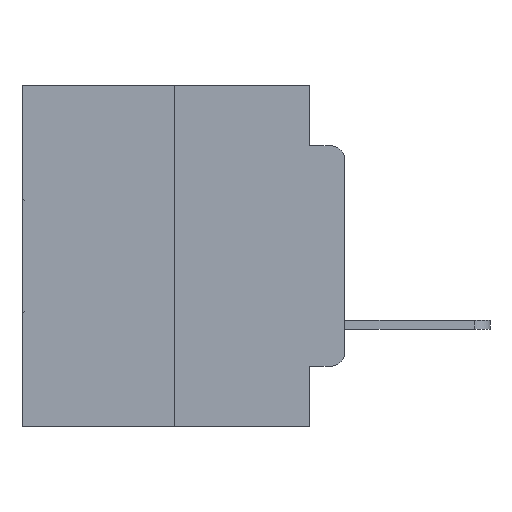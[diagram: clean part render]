
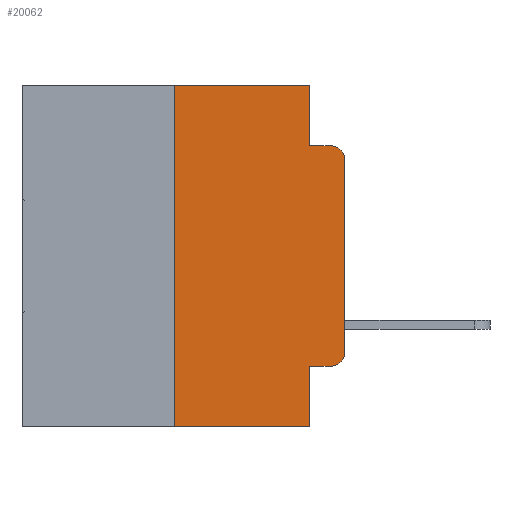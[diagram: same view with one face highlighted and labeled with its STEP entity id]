
A CAD part, left-side view. The second image highlights one B-rep face of the part: STEP entity #20062.
In plain terms, the highlighted planar face has unit normal (-1, 0, 0).
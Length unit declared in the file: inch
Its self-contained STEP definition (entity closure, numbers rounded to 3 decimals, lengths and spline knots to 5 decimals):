
#60 = CARTESIAN_POINT ( 'NONE',  ( 0., 0.051, -0.0885 ) ) ;
#157 = CARTESIAN_POINT ( 'NONE',  ( 0., 0.02, -0.3915 ) ) ;
#269 = ORIENTED_EDGE ( 'NONE', *, *, #30994, .F. ) ;
#780 = LINE ( 'NONE', #2235, #20785 ) ;
#942 = CARTESIAN_POINT ( 'NONE',  ( 0., 0., -0.1085 ) ) ;
#957 = ORIENTED_EDGE ( 'NONE', *, *, #22711, .T. ) ;
#1211 = ORIENTED_EDGE ( 'NONE', *, *, #21705, .T. ) ;
#1586 = VECTOR ( 'NONE', #13618, 39.37008 ) ;
#1912 = VERTEX_POINT ( 'NONE', #25877 ) ;
#2235 = CARTESIAN_POINT ( 'NONE',  ( 0., 0.051, -0.4115 ) ) ;
#2318 = EDGE_CURVE ( 'NONE', #24108, #1912, #25616, .T. ) ;
#2443 = VECTOR ( 'NONE', #11772, 39.37008 ) ;
#2888 = DIRECTION ( 'NONE',  ( 0., 0., -1. ) ) ;
#3229 = CARTESIAN_POINT ( 'NONE',  ( 0., 0.02, -0.4115 ) ) ;
#3247 = LINE ( 'NONE', #16661, #28120 ) ;
#4079 = VECTOR ( 'NONE', #18414, 39.37008 ) ;
#4267 = EDGE_CURVE ( 'NONE', #18400, #5257, #29438, .T. ) ;
#5257 = VERTEX_POINT ( 'NONE', #10855 ) ;
#5458 = CARTESIAN_POINT ( 'NONE',  ( 0., 0.051, -0.4115 ) ) ;
#5983 = PLANE ( 'NONE',  #12630 ) ;
#6089 = AXIS2_PLACEMENT_3D ( 'NONE', #24161, #29414, #29419 ) ;
#6649 = VECTOR ( 'NONE', #28422, 39.37008 ) ;
#6708 = CARTESIAN_POINT ( 'NONE',  ( 0., 0., -0.3915 ) ) ;
#7072 = CARTESIAN_POINT ( 'NONE',  ( 0., 0.25, -0.5 ) ) ;
#7137 = CARTESIAN_POINT ( 'NONE',  ( 0., 0.051, -0.0885 ) ) ;
#7579 = VERTEX_POINT ( 'NONE', #5458 ) ;
#7783 = AXIS2_PLACEMENT_3D ( 'NONE', #157, #18038, #2888 ) ;
#8531 = DIRECTION ( 'NONE',  ( 0., 0., -1. ) ) ;
#8793 = VERTEX_POINT ( 'NONE', #6708 ) ;
#10855 = CARTESIAN_POINT ( 'NONE',  ( 0., 0.25, 0. ) ) ;
#11091 = DIRECTION ( 'NONE',  ( 0., 0., -1. ) ) ;
#11772 = DIRECTION ( 'NONE',  ( 0., -1., 0. ) ) ;
#12368 = VERTEX_POINT ( 'NONE', #21051 ) ;
#12630 = AXIS2_PLACEMENT_3D ( 'NONE', #22774, #25169, #11091 ) ;
#13618 = DIRECTION ( 'NONE',  ( 0., 0., 1. ) ) ;
#13876 = LINE ( 'NONE', #16652, #19439 ) ;
#14248 = DIRECTION ( 'NONE',  ( 0., 0., -1. ) ) ;
#15031 = EDGE_CURVE ( 'NONE', #17494, #1912, #26417, .T. ) ;
#16448 = EDGE_CURVE ( 'NONE', #12368, #17494, #3247, .T. ) ;
#16652 = CARTESIAN_POINT ( 'NONE',  ( 0., 0.473, 0. ) ) ;
#16661 = CARTESIAN_POINT ( 'NONE',  ( 0., 0.051, 0. ) ) ;
#17494 = VERTEX_POINT ( 'NONE', #60 ) ;
#17636 = EDGE_LOOP ( 'NONE', ( #18782, #19552, #21857, #22356, #22534, #23887, #26250, #269, #957, #1211 ) ) ;
#18038 = DIRECTION ( 'NONE',  ( -1., 0., 0. ) ) ;
#18062 = EDGE_CURVE ( 'NONE', #8793, #24108, #31083, .T. ) ;
#18400 = VERTEX_POINT ( 'NONE', #7072 ) ;
#18414 = DIRECTION ( 'NONE',  ( 0., 0., 1. ) ) ;
#18616 = CARTESIAN_POINT ( 'NONE',  ( 0., 0.25, 0. ) ) ;
#18782 = ORIENTED_EDGE ( 'NONE', *, *, #18062, .T. ) ;
#18918 = CARTESIAN_POINT ( 'NONE',  ( 0., 0.051, -0.5 ) ) ;
#19439 = VECTOR ( 'NONE', #25855, 39.37008 ) ;
#19552 = ORIENTED_EDGE ( 'NONE', *, *, #2318, .T. ) ;
#19797 = CIRCLE ( 'NONE', #7783, 0.02 ) ;
#20062 = ADVANCED_FACE ( 'NONE', ( #20958 ), #5983, .F. ) ;
#20069 = VERTEX_POINT ( 'NONE', #3229 ) ;
#20231 = VERTEX_POINT ( 'NONE', #18918 ) ;
#20785 = VECTOR ( 'NONE', #21933, 39.37008 ) ;
#20958 = FACE_OUTER_BOUND ( 'NONE', #17636, .T. ) ;
#21051 = CARTESIAN_POINT ( 'NONE',  ( 0., 0.051, 0. ) ) ;
#21208 = CARTESIAN_POINT ( 'NONE',  ( 0., 0.473, -0.5 ) ) ;
#21705 = EDGE_CURVE ( 'NONE', #20069, #8793, #19797, .T. ) ;
#21857 = ORIENTED_EDGE ( 'NONE', *, *, #15031, .F. ) ;
#21933 = DIRECTION ( 'NONE',  ( 0., -1., 0. ) ) ;
#22356 = ORIENTED_EDGE ( 'NONE', *, *, #16448, .F. ) ;
#22534 = ORIENTED_EDGE ( 'NONE', *, *, #26894, .F. ) ;
#22638 = CARTESIAN_POINT ( 'NONE',  ( 0., 0.051, 0. ) ) ;
#22711 = EDGE_CURVE ( 'NONE', #7579, #20069, #780, .T. ) ;
#22774 = CARTESIAN_POINT ( 'NONE',  ( 0., 0.473, 0. ) ) ;
#23025 = VECTOR ( 'NONE', #8531, 39.37008 ) ;
#23887 = ORIENTED_EDGE ( 'NONE', *, *, #4267, .F. ) ;
#24108 = VERTEX_POINT ( 'NONE', #942 ) ;
#24161 = CARTESIAN_POINT ( 'NONE',  ( 0., 0.02, -0.1085 ) ) ;
#25169 = DIRECTION ( 'NONE',  ( 1., 0., 0. ) ) ;
#25616 = CIRCLE ( 'NONE', #6089, 0.02 ) ;
#25855 = DIRECTION ( 'NONE',  ( 0., -1., 0. ) ) ;
#25877 = CARTESIAN_POINT ( 'NONE',  ( 0., 0.02, -0.0885 ) ) ;
#26250 = ORIENTED_EDGE ( 'NONE', *, *, #28133, .T. ) ;
#26417 = LINE ( 'NONE', #7137, #6649 ) ;
#26894 = EDGE_CURVE ( 'NONE', #5257, #12368, #13876, .T. ) ;
#27439 = CARTESIAN_POINT ( 'NONE',  ( 0., 0., 0. ) ) ;
#27493 = LINE ( 'NONE', #21208, #2443 ) ;
#28120 = VECTOR ( 'NONE', #14248, 39.37008 ) ;
#28133 = EDGE_CURVE ( 'NONE', #18400, #20231, #27493, .T. ) ;
#28422 = DIRECTION ( 'NONE',  ( 0., -1., 0. ) ) ;
#28980 = LINE ( 'NONE', #22638, #23025 ) ;
#29414 = DIRECTION ( 'NONE',  ( -1., 0., 0. ) ) ;
#29419 = DIRECTION ( 'NONE',  ( 0., 0., -1. ) ) ;
#29438 = LINE ( 'NONE', #18616, #4079 ) ;
#30994 = EDGE_CURVE ( 'NONE', #7579, #20231, #28980, .T. ) ;
#31083 = LINE ( 'NONE', #27439, #1586 ) ;
